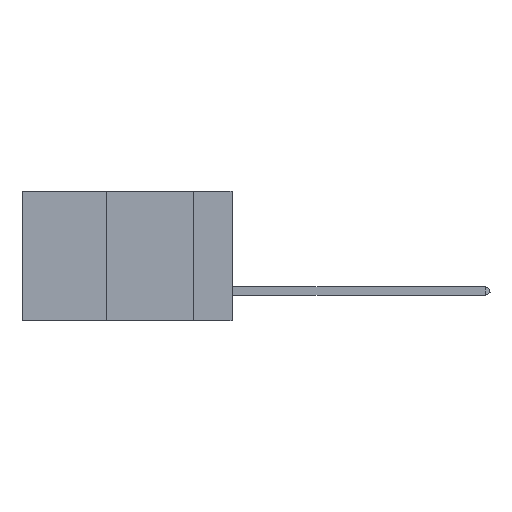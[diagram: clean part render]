
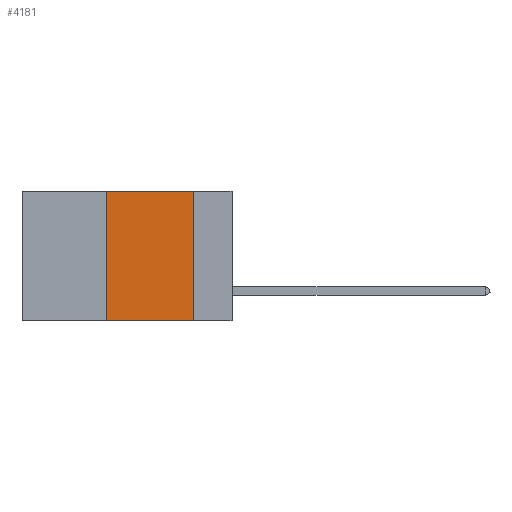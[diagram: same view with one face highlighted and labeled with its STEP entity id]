
A CAD part, left-side view. The second image highlights one B-rep face of the part: STEP entity #4181.
In plain terms, the highlighted planar face has unit normal (-1, 0, 0).
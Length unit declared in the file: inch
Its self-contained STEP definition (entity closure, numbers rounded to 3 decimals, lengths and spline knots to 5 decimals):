
#376 = EDGE_LOOP ( 'NONE', ( #15074, #11324, #20507, #7079 ) ) ;
#601 = CARTESIAN_POINT ( 'NONE',  ( 0., 0.11, 0. ) ) ;
#967 = VERTEX_POINT ( 'NONE', #601 ) ;
#1297 = DIRECTION ( 'NONE',  ( 0., 0., -1. ) ) ;
#1404 = DIRECTION ( 'NONE',  ( 1., 0., 0. ) ) ;
#3169 = AXIS2_PLACEMENT_3D ( 'NONE', #6321, #1404, #1297 ) ;
#4181 = ADVANCED_FACE ( 'NONE', ( #9736 ), #5819, .F. ) ;
#4865 = VECTOR ( 'NONE', #12528, 39.37008 ) ;
#5819 = PLANE ( 'NONE',  #3169 ) ;
#6085 = CARTESIAN_POINT ( 'NONE',  ( 0., 0.6, 0. ) ) ;
#6232 = DIRECTION ( 'NONE',  ( 0., -1., 0. ) ) ;
#6321 = CARTESIAN_POINT ( 'NONE',  ( 0., 0.6, 0. ) ) ;
#6427 = DIRECTION ( 'NONE',  ( 0., 0., -1. ) ) ;
#6692 = EDGE_CURVE ( 'NONE', #17793, #15831, #15718, .T. ) ;
#7079 = ORIENTED_EDGE ( 'NONE', *, *, #17466, .T. ) ;
#7481 = DIRECTION ( 'NONE',  ( 0., -1., 0. ) ) ;
#7632 = CARTESIAN_POINT ( 'NONE',  ( 0., 0.36, 0. ) ) ;
#8710 = CARTESIAN_POINT ( 'NONE',  ( 0., 0.36, 0. ) ) ;
#9736 = FACE_OUTER_BOUND ( 'NONE', #376, .T. ) ;
#10494 = CARTESIAN_POINT ( 'NONE',  ( 0., 0.36, -0.37 ) ) ;
#11248 = CARTESIAN_POINT ( 'NONE',  ( 0., 0.6, -0.37 ) ) ;
#11324 = ORIENTED_EDGE ( 'NONE', *, *, #13470, .F. ) ;
#12528 = DIRECTION ( 'NONE',  ( 0., 0., 1. ) ) ;
#12729 = LINE ( 'NONE', #11248, #18892 ) ;
#13021 = LINE ( 'NONE', #16227, #16239 ) ;
#13126 = EDGE_CURVE ( 'NONE', #967, #16282, #13021, .T. ) ;
#13470 = EDGE_CURVE ( 'NONE', #15831, #967, #14179, .T. ) ;
#14179 = LINE ( 'NONE', #6085, #15915 ) ;
#15074 = ORIENTED_EDGE ( 'NONE', *, *, #13126, .F. ) ;
#15718 = LINE ( 'NONE', #7632, #4865 ) ;
#15831 = VERTEX_POINT ( 'NONE', #8710 ) ;
#15915 = VECTOR ( 'NONE', #7481, 39.37008 ) ;
#16227 = CARTESIAN_POINT ( 'NONE',  ( 0., 0.11, 0. ) ) ;
#16239 = VECTOR ( 'NONE', #6427, 39.37008 ) ;
#16282 = VERTEX_POINT ( 'NONE', #17276 ) ;
#17276 = CARTESIAN_POINT ( 'NONE',  ( 0., 0.11, -0.37 ) ) ;
#17466 = EDGE_CURVE ( 'NONE', #17793, #16282, #12729, .T. ) ;
#17793 = VERTEX_POINT ( 'NONE', #10494 ) ;
#18892 = VECTOR ( 'NONE', #6232, 39.37008 ) ;
#20507 = ORIENTED_EDGE ( 'NONE', *, *, #6692, .F. ) ;
